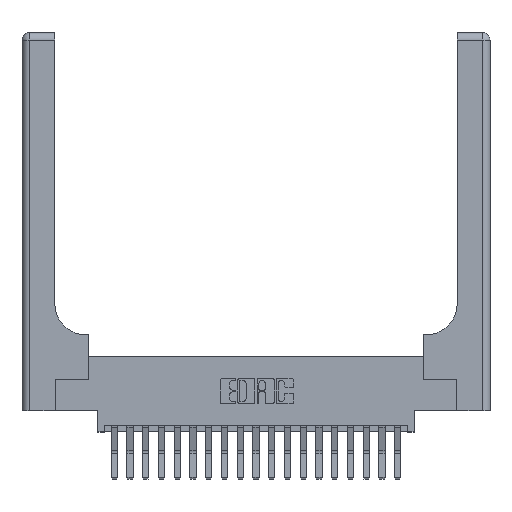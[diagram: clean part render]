
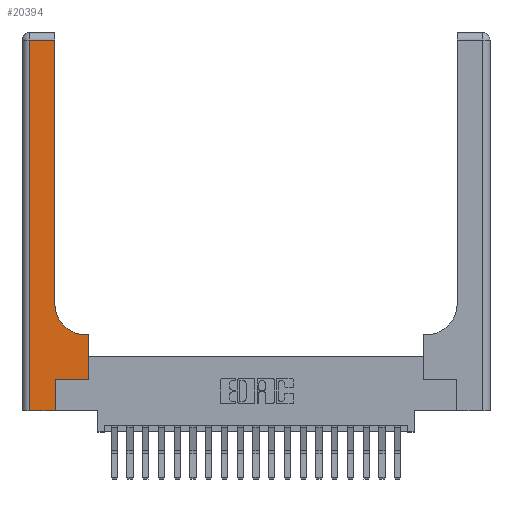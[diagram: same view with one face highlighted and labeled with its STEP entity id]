
A CAD part, top view. The second image highlights one B-rep face of the part: STEP entity #20394.
In plain terms, the highlighted planar face has unit normal (0, 0, 1).
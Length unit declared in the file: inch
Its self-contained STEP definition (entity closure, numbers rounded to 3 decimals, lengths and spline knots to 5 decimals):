
#92 = CARTESIAN_POINT ( 'NONE',  ( 0.528, 0.25, 0.37 ) ) ;
#314 = CARTESIAN_POINT ( 'NONE',  ( 0.06, 0., 0.37 ) ) ;
#939 = LINE ( 'NONE', #3844, #15329 ) ;
#1044 = DIRECTION ( 'NONE',  ( 1., 0., 0. ) ) ;
#1091 = CARTESIAN_POINT ( 'NONE',  ( 0.528, 0.6, 0.37 ) ) ;
#1535 = EDGE_CURVE ( 'NONE', #12261, #9398, #4897, .T. ) ;
#1593 = EDGE_CURVE ( 'NONE', #17862, #12261, #8187, .T. ) ;
#2395 = CARTESIAN_POINT ( 'NONE',  ( 0., 2.94, 0.37 ) ) ;
#2831 = LINE ( 'NONE', #10206, #10430 ) ;
#2946 = AXIS2_PLACEMENT_3D ( 'NONE', #4758, #15959, #6390 ) ;
#3548 = VERTEX_POINT ( 'NONE', #314 ) ;
#3574 = FACE_OUTER_BOUND ( 'NONE', #9662, .T. ) ;
#3844 = CARTESIAN_POINT ( 'NONE',  ( 0.265, 0., 0.37 ) ) ;
#4064 = DIRECTION ( 'NONE',  ( -1., 0., 0. ) ) ;
#4619 = CARTESIAN_POINT ( 'NONE',  ( 0.528, 0.25, 0.37 ) ) ;
#4700 = VERTEX_POINT ( 'NONE', #6837 ) ;
#4733 = EDGE_CURVE ( 'NONE', #6988, #13341, #10993, .T. ) ;
#4758 = CARTESIAN_POINT ( 'NONE',  ( 0., 3., 0.37 ) ) ;
#4897 = LINE ( 'NONE', #9353, #12949 ) ;
#4957 = DIRECTION ( 'NONE',  ( 0., -1., 0. ) ) ;
#5232 = CARTESIAN_POINT ( 'NONE',  ( 0.26, 2.94, 0.37 ) ) ;
#5339 = CARTESIAN_POINT ( 'NONE',  ( 0.26, 3., 0.37 ) ) ;
#5801 = ORIENTED_EDGE ( 'NONE', *, *, #1535, .T. ) ;
#5989 = ORIENTED_EDGE ( 'NONE', *, *, #12023, .T. ) ;
#6079 = CARTESIAN_POINT ( 'NONE',  ( 0.06, 2.94, 0.37 ) ) ;
#6255 = DIRECTION ( 'NONE',  ( 0., 1., 0. ) ) ;
#6390 = DIRECTION ( 'NONE',  ( -1., 0., 0. ) ) ;
#6558 = DIRECTION ( 'NONE',  ( 1., 0., 0. ) ) ;
#6837 = CARTESIAN_POINT ( 'NONE',  ( 0.265, 0., 0.37 ) ) ;
#6988 = VERTEX_POINT ( 'NONE', #7801 ) ;
#7111 = VERTEX_POINT ( 'NONE', #16736 ) ;
#7801 = CARTESIAN_POINT ( 'NONE',  ( 0.26, 0.85, 0.37 ) ) ;
#7854 = ORIENTED_EDGE ( 'NONE', *, *, #8953, .T. ) ;
#7909 = VERTEX_POINT ( 'NONE', #6079 ) ;
#8187 = LINE ( 'NONE', #4619, #16163 ) ;
#8358 = CARTESIAN_POINT ( 'NONE',  ( 0.51, 0.6, 0.37 ) ) ;
#8625 = EDGE_CURVE ( 'NONE', #7111, #17862, #20614, .T. ) ;
#8953 = EDGE_CURVE ( 'NONE', #13341, #7909, #15058, .T. ) ;
#8989 = LINE ( 'NONE', #14364, #10499 ) ;
#9353 = CARTESIAN_POINT ( 'NONE',  ( 0.26, 0.6, 0.37 ) ) ;
#9398 = VERTEX_POINT ( 'NONE', #8358 ) ;
#9662 = EDGE_LOOP ( 'NONE', ( #17518, #7854, #20790, #10846, #5989, #18333, #20116, #5801, #20809 ) ) ;
#10206 = CARTESIAN_POINT ( 'NONE',  ( 0., 0., 0.37 ) ) ;
#10275 = EDGE_CURVE ( 'NONE', #3548, #4700, #2831, .T. ) ;
#10430 = VECTOR ( 'NONE', #13339, 39.37008 ) ;
#10499 = VECTOR ( 'NONE', #4957, 39.37008 ) ;
#10666 = AXIS2_PLACEMENT_3D ( 'NONE', #20354, #10780, #1044 ) ;
#10780 = DIRECTION ( 'NONE',  ( 0., 0., -1. ) ) ;
#10846 = ORIENTED_EDGE ( 'NONE', *, *, #10275, .T. ) ;
#10984 = DIRECTION ( 'NONE',  ( -1., 0., 0. ) ) ;
#10993 = LINE ( 'NONE', #5339, #11507 ) ;
#11507 = VECTOR ( 'NONE', #16522, 39.37008 ) ;
#12023 = EDGE_CURVE ( 'NONE', #4700, #7111, #939, .T. ) ;
#12261 = VERTEX_POINT ( 'NONE', #1091 ) ;
#12949 = VECTOR ( 'NONE', #10984, 39.37008 ) ;
#13339 = DIRECTION ( 'NONE',  ( 1., 0., 0. ) ) ;
#13341 = VERTEX_POINT ( 'NONE', #5232 ) ;
#14364 = CARTESIAN_POINT ( 'NONE',  ( 0.06, 3., 0.37 ) ) ;
#14380 = PLANE ( 'NONE',  #2946 ) ;
#14842 = EDGE_CURVE ( 'NONE', #7909, #3548, #8989, .T. ) ;
#15058 = LINE ( 'NONE', #2395, #18820 ) ;
#15329 = VECTOR ( 'NONE', #19858, 39.37008 ) ;
#15959 = DIRECTION ( 'NONE',  ( 0., 0., -1. ) ) ;
#16163 = VECTOR ( 'NONE', #6255, 39.37008 ) ;
#16522 = DIRECTION ( 'NONE',  ( 0., 1., 0. ) ) ;
#16736 = CARTESIAN_POINT ( 'NONE',  ( 0.265, 0.25, 0.37 ) ) ;
#16816 = VECTOR ( 'NONE', #6558, 39.37008 ) ;
#17518 = ORIENTED_EDGE ( 'NONE', *, *, #4733, .T. ) ;
#17720 = CARTESIAN_POINT ( 'NONE',  ( 0.265, 0.25, 0.37 ) ) ;
#17862 = VERTEX_POINT ( 'NONE', #92 ) ;
#18333 = ORIENTED_EDGE ( 'NONE', *, *, #8625, .T. ) ;
#18390 = CIRCLE ( 'NONE', #10666, 0.25 ) ;
#18820 = VECTOR ( 'NONE', #4064, 39.37008 ) ;
#19721 = EDGE_CURVE ( 'NONE', #9398, #6988, #18390, .T. ) ;
#19858 = DIRECTION ( 'NONE',  ( 0., 1., 0. ) ) ;
#20116 = ORIENTED_EDGE ( 'NONE', *, *, #1593, .T. ) ;
#20354 = CARTESIAN_POINT ( 'NONE',  ( 0.51, 0.85, 0.37 ) ) ;
#20394 = ADVANCED_FACE ( 'NONE', ( #3574 ), #14380, .F. ) ;
#20614 = LINE ( 'NONE', #17720, #16816 ) ;
#20790 = ORIENTED_EDGE ( 'NONE', *, *, #14842, .T. ) ;
#20809 = ORIENTED_EDGE ( 'NONE', *, *, #19721, .T. ) ;
